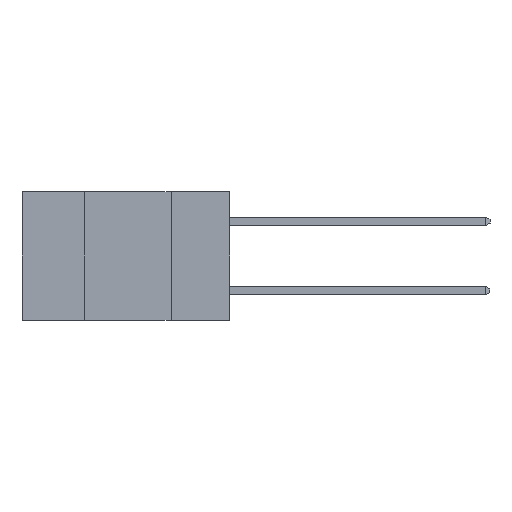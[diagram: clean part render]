
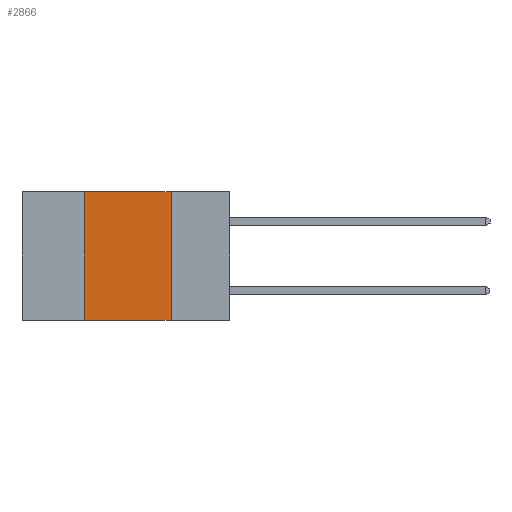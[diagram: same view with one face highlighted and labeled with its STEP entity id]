
A CAD part, left-side view. The second image highlights one B-rep face of the part: STEP entity #2866.
In plain terms, the highlighted planar face has unit normal (-1, 0, 0).
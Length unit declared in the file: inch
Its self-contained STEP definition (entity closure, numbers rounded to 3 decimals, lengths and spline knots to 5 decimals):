
#76 = EDGE_LOOP ( 'NONE', ( #577, #792, #961, #1028 ) ) ;
#152 = LINE ( 'NONE', #9008, #7773 ) ;
#377 = VERTEX_POINT ( 'NONE', #8410 ) ;
#471 = VECTOR ( 'NONE', #4827, 39.37008 ) ;
#549 = EDGE_CURVE ( 'NONE', #4556, #4972, #2783, .T. ) ;
#577 = ORIENTED_EDGE ( 'NONE', *, *, #5457, .F. ) ;
#650 = FACE_OUTER_BOUND ( 'NONE', #76, .T. ) ;
#674 = DIRECTION ( 'NONE',  ( 0., 0., -1. ) ) ;
#792 = ORIENTED_EDGE ( 'NONE', *, *, #549, .F. ) ;
#961 = ORIENTED_EDGE ( 'NONE', *, *, #5496, .F. ) ;
#1028 = ORIENTED_EDGE ( 'NONE', *, *, #5636, .T. ) ;
#2248 = CARTESIAN_POINT ( 'NONE',  ( 0., 0.6, 0. ) ) ;
#2727 = VERTEX_POINT ( 'NONE', #7109 ) ;
#2783 = LINE ( 'NONE', #2248, #471 ) ;
#2866 = ADVANCED_FACE ( 'NONE', ( #650 ), #8954, .F. ) ;
#4224 = LINE ( 'NONE', #9027, #7677 ) ;
#4422 = CARTESIAN_POINT ( 'NONE',  ( 0., 0.17, 0. ) ) ;
#4556 = VERTEX_POINT ( 'NONE', #6554 ) ;
#4827 = DIRECTION ( 'NONE',  ( 0., -1., 0. ) ) ;
#4972 = VERTEX_POINT ( 'NONE', #4422 ) ;
#5457 = EDGE_CURVE ( 'NONE', #4972, #377, #4224, .T. ) ;
#5496 = EDGE_CURVE ( 'NONE', #2727, #4556, #7318, .T. ) ;
#5636 = EDGE_CURVE ( 'NONE', #2727, #377, #152, .T. ) ;
#5674 = AXIS2_PLACEMENT_3D ( 'NONE', #6769, #7844, #9127 ) ;
#6196 = DIRECTION ( 'NONE',  ( 0., 0., 1. ) ) ;
#6554 = CARTESIAN_POINT ( 'NONE',  ( 0., 0.42, 0. ) ) ;
#6769 = CARTESIAN_POINT ( 'NONE',  ( 0., 0.6, 0. ) ) ;
#7109 = CARTESIAN_POINT ( 'NONE',  ( 0., 0.42, -0.37 ) ) ;
#7318 = LINE ( 'NONE', #9175, #8727 ) ;
#7554 = DIRECTION ( 'NONE',  ( 0., -1., 0. ) ) ;
#7677 = VECTOR ( 'NONE', #674, 39.37008 ) ;
#7773 = VECTOR ( 'NONE', #7554, 39.37008 ) ;
#7844 = DIRECTION ( 'NONE',  ( 1., 0., 0. ) ) ;
#8410 = CARTESIAN_POINT ( 'NONE',  ( 0., 0.17, -0.37 ) ) ;
#8727 = VECTOR ( 'NONE', #6196, 39.37008 ) ;
#8954 = PLANE ( 'NONE',  #5674 ) ;
#9008 = CARTESIAN_POINT ( 'NONE',  ( 0., 0.6, -0.37 ) ) ;
#9027 = CARTESIAN_POINT ( 'NONE',  ( 0., 0.17, 0. ) ) ;
#9127 = DIRECTION ( 'NONE',  ( 0., 0., -1. ) ) ;
#9175 = CARTESIAN_POINT ( 'NONE',  ( 0., 0.42, 0. ) ) ;
